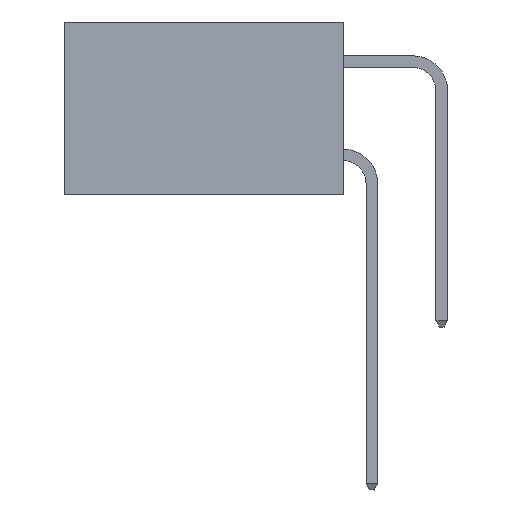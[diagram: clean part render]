
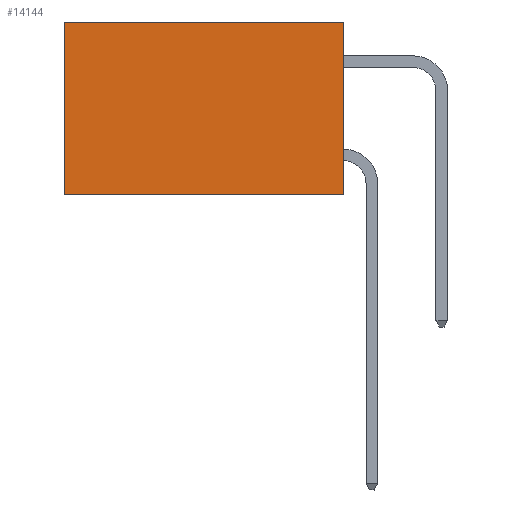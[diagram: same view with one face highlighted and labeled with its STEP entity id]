
A CAD part, left-side view. The second image highlights one B-rep face of the part: STEP entity #14144.
In plain terms, the highlighted planar face has unit normal (-1, 0, 0).
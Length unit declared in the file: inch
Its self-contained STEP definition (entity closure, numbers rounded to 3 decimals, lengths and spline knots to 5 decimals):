
#1226 = EDGE_LOOP ( 'NONE', ( #4062, #13678, #18361, #11816 ) ) ;
#1857 = CARTESIAN_POINT ( 'NONE',  ( 0.2615, 0.6, -0.37 ) ) ;
#2629 = VERTEX_POINT ( 'NONE', #4525 ) ;
#3720 = DIRECTION ( 'NONE',  ( 0., 1., 0. ) ) ;
#3778 = VECTOR ( 'NONE', #3720, 39.37008 ) ;
#4062 = ORIENTED_EDGE ( 'NONE', *, *, #8517, .T. ) ;
#4525 = CARTESIAN_POINT ( 'NONE',  ( 0.2615, 0., 0. ) ) ;
#5708 = FACE_OUTER_BOUND ( 'NONE', #1226, .T. ) ;
#5786 = CARTESIAN_POINT ( 'NONE',  ( 0.2615, 0., -0.37 ) ) ;
#5988 = VERTEX_POINT ( 'NONE', #17648 ) ;
#6731 = CARTESIAN_POINT ( 'NONE',  ( 0.2615, 0.6, 0. ) ) ;
#6803 = AXIS2_PLACEMENT_3D ( 'NONE', #14422, #22774, #16074 ) ;
#7117 = VECTOR ( 'NONE', #26181, 39.37008 ) ;
#7418 = LINE ( 'NONE', #18051, #7117 ) ;
#8517 = EDGE_CURVE ( 'NONE', #19180, #25209, #10189, .T. ) ;
#9877 = LINE ( 'NONE', #5786, #3778 ) ;
#10189 = LINE ( 'NONE', #1857, #12091 ) ;
#10370 = LINE ( 'NONE', #18695, #26075 ) ;
#11816 = ORIENTED_EDGE ( 'NONE', *, *, #13023, .T. ) ;
#12091 = VECTOR ( 'NONE', #18128, 39.37008 ) ;
#13023 = EDGE_CURVE ( 'NONE', #2629, #19180, #7418, .T. ) ;
#13678 = ORIENTED_EDGE ( 'NONE', *, *, #17708, .F. ) ;
#14144 = ADVANCED_FACE ( 'NONE', ( #5708 ), #24319, .F. ) ;
#14338 = DIRECTION ( 'NONE',  ( 0., 0., -1. ) ) ;
#14422 = CARTESIAN_POINT ( 'NONE',  ( 0.2615, 0., -0.37 ) ) ;
#16074 = DIRECTION ( 'NONE',  ( 0., 0., -1. ) ) ;
#16904 = EDGE_CURVE ( 'NONE', #2629, #5988, #10370, .T. ) ;
#17614 = CARTESIAN_POINT ( 'NONE',  ( 0.2615, 0.6, -0.37 ) ) ;
#17648 = CARTESIAN_POINT ( 'NONE',  ( 0.2615, 0., -0.37 ) ) ;
#17708 = EDGE_CURVE ( 'NONE', #5988, #25209, #9877, .T. ) ;
#18051 = CARTESIAN_POINT ( 'NONE',  ( 0.2615, 0., 0. ) ) ;
#18128 = DIRECTION ( 'NONE',  ( 0., 0., -1. ) ) ;
#18361 = ORIENTED_EDGE ( 'NONE', *, *, #16904, .F. ) ;
#18695 = CARTESIAN_POINT ( 'NONE',  ( 0.2615, 0., -0.37 ) ) ;
#19180 = VERTEX_POINT ( 'NONE', #6731 ) ;
#22774 = DIRECTION ( 'NONE',  ( 1., 0., 0. ) ) ;
#24319 = PLANE ( 'NONE',  #6803 ) ;
#25209 = VERTEX_POINT ( 'NONE', #17614 ) ;
#26075 = VECTOR ( 'NONE', #14338, 39.37008 ) ;
#26181 = DIRECTION ( 'NONE',  ( 0., 1., 0. ) ) ;
